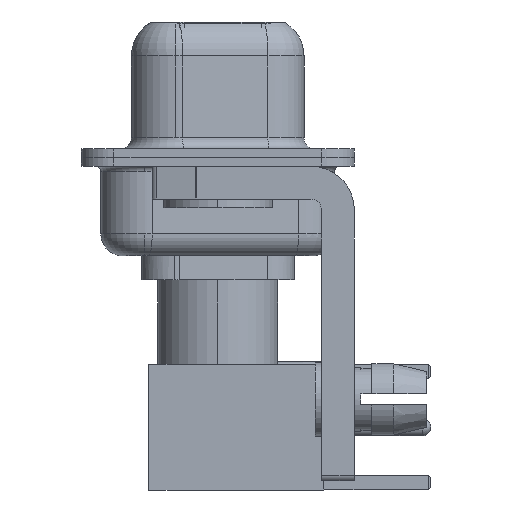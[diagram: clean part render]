
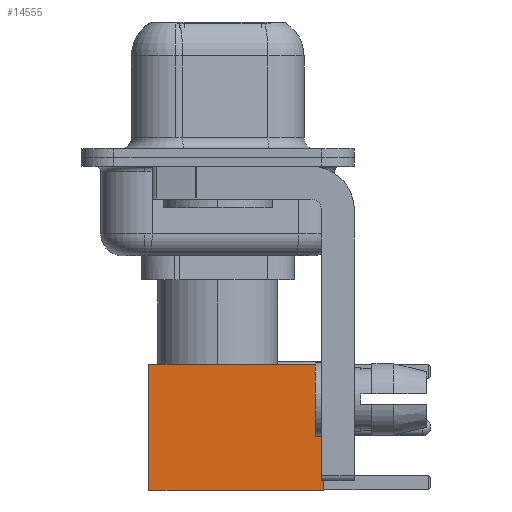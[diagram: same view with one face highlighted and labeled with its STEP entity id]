
A CAD part, left-side view. The second image highlights one B-rep face of the part: STEP entity #14555.
In plain terms, the highlighted face is planar.
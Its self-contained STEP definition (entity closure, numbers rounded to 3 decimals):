
#1143 = CARTESIAN_POINT ( 'NONE',  ( 2.875, 2.875, 0. ) ) ;
#2063 = LINE ( 'NONE', #11312, #29794 ) ;
#3638 = VECTOR ( 'NONE', #5173, 1000. ) ;
#5173 = DIRECTION ( 'NONE',  ( -1., 0., 0. ) ) ;
#6277 = LINE ( 'NONE', #1143, #17494 ) ;
#6642 = FACE_OUTER_BOUND ( 'NONE', #6706, .T. ) ;
#6706 = EDGE_LOOP ( 'NONE', ( #19172, #18358, #6838, #25444 ) ) ;
#6838 = ORIENTED_EDGE ( 'NONE', *, *, #19431, .F. ) ;
#7101 = VERTEX_POINT ( 'NONE', #26192 ) ;
#10234 = DIRECTION ( 'NONE',  ( 0., 0., -1. ) ) ;
#10804 = AXIS2_PLACEMENT_3D ( 'NONE', #22857, #29448, #29755 ) ;
#11071 = VERTEX_POINT ( 'NONE', #28267 ) ;
#11312 = CARTESIAN_POINT ( 'NONE',  ( -2.875, 2.875, 0. ) ) ;
#11696 = CARTESIAN_POINT ( 'NONE',  ( 0., 2.875, 8. ) ) ;
#14296 = LINE ( 'NONE', #11696, #3638 ) ;
#14555 = ADVANCED_FACE ( 'NONE', ( #6642 ), #27036, .T. ) ;
#15710 = DIRECTION ( 'NONE',  ( -1., 0., 0. ) ) ;
#17494 = VECTOR ( 'NONE', #10234, 1000. ) ;
#17829 = CARTESIAN_POINT ( 'NONE',  ( 0., 2.875, 0. ) ) ;
#17979 = LINE ( 'NONE', #17829, #21134 ) ;
#18296 = DIRECTION ( 'NONE',  ( 0., 0., -1. ) ) ;
#18358 = ORIENTED_EDGE ( 'NONE', *, *, #27285, .T. ) ;
#19172 = ORIENTED_EDGE ( 'NONE', *, *, #21142, .T. ) ;
#19431 = EDGE_CURVE ( 'NONE', #7101, #21201, #2063, .T. ) ;
#20756 = VERTEX_POINT ( 'NONE', #22996 ) ;
#21134 = VECTOR ( 'NONE', #15710, 1000. ) ;
#21142 = EDGE_CURVE ( 'NONE', #20756, #11071, #6277, .T. ) ;
#21201 = VERTEX_POINT ( 'NONE', #22191 ) ;
#22191 = CARTESIAN_POINT ( 'NONE',  ( -2.875, 2.875, 0. ) ) ;
#22857 = CARTESIAN_POINT ( 'NONE',  ( 2.875, 2.875, 0. ) ) ;
#22996 = CARTESIAN_POINT ( 'NONE',  ( 2.875, 2.875, 8. ) ) ;
#25034 = EDGE_CURVE ( 'NONE', #20756, #7101, #14296, .T. ) ;
#25444 = ORIENTED_EDGE ( 'NONE', *, *, #25034, .F. ) ;
#26192 = CARTESIAN_POINT ( 'NONE',  ( -2.875, 2.875, 8. ) ) ;
#27036 = PLANE ( 'NONE',  #10804 ) ;
#27285 = EDGE_CURVE ( 'NONE', #11071, #21201, #17979, .T. ) ;
#28267 = CARTESIAN_POINT ( 'NONE',  ( 2.875, 2.875, 0. ) ) ;
#29448 = DIRECTION ( 'NONE',  ( 0., 1., 0. ) ) ;
#29755 = DIRECTION ( 'NONE',  ( 0., 0., 1. ) ) ;
#29794 = VECTOR ( 'NONE', #18296, 1000. ) ;
